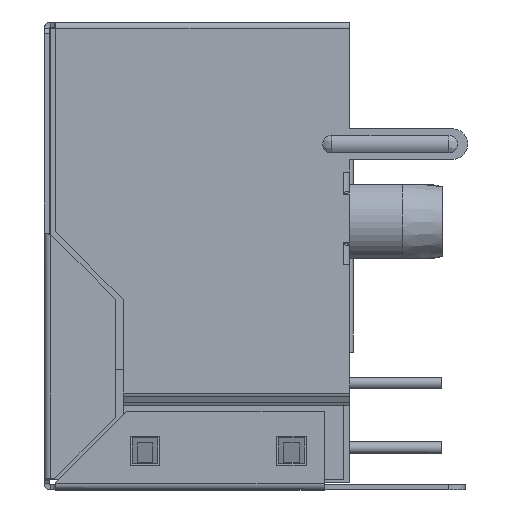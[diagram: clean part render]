
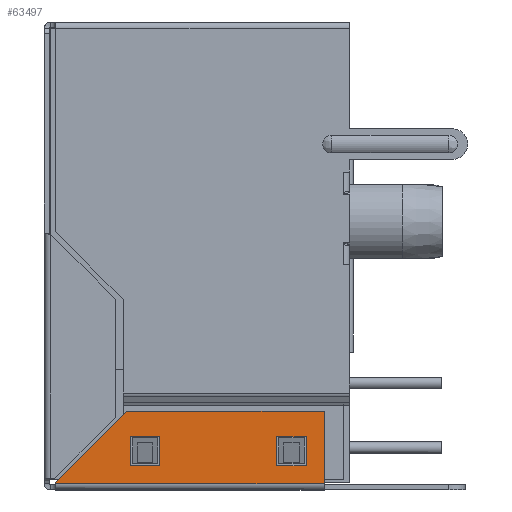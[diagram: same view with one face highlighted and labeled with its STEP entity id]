
A CAD part, left-side view. The second image highlights one B-rep face of the part: STEP entity #63497.
In plain terms, the highlighted planar face has unit normal (-1, 0, 0).
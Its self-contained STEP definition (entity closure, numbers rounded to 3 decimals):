
#437 = LINE ( 'NONE', #15104, #49154 ) ;
#512 = LINE ( 'NONE', #66749, #61142 ) ;
#621 = ORIENTED_EDGE ( 'NONE', *, *, #53207, .T. ) ;
#1085 = VECTOR ( 'NONE', #66073, 1000. ) ;
#2873 = DIRECTION ( 'NONE',  ( 0., 0.707, -0.707 ) ) ;
#2953 = DIRECTION ( 'NONE',  ( -1., 0., 0. ) ) ;
#3156 = CARTESIAN_POINT ( 'NONE',  ( -29.5, -3.145, -8.251 ) ) ;
#3959 = FACE_BOUND ( 'NONE', #29592, .T. ) ;
#4478 = VERTEX_POINT ( 'NONE', #22803 ) ;
#4897 = CARTESIAN_POINT ( 'NONE',  ( -29.5, 5.543, -8.951 ) ) ;
#5461 = LINE ( 'NONE', #19885, #10014 ) ;
#6989 = CARTESIAN_POINT ( 'NONE',  ( -29.5, 2.605, -8.251 ) ) ;
#9413 = ORIENTED_EDGE ( 'NONE', *, *, #43607, .T. ) ;
#9445 = ORIENTED_EDGE ( 'NONE', *, *, #21681, .F. ) ;
#9524 = CARTESIAN_POINT ( 'NONE',  ( -29.5, -5.211, -8.251 ) ) ;
#9581 = DIRECTION ( 'NONE',  ( 0., 0., -1. ) ) ;
#9731 = FACE_BOUND ( 'NONE', #72329, .T. ) ;
#10014 = VECTOR ( 'NONE', #50106, 1000. ) ;
#10704 = EDGE_CURVE ( 'NONE', #52799, #46683, #71140, .T. ) ;
#11021 = DIRECTION ( 'NONE',  ( 0., -1., 0. ) ) ;
#12224 = DIRECTION ( 'NONE',  ( 0., 1., 0. ) ) ;
#12351 = EDGE_CURVE ( 'NONE', #4478, #56018, #74597, .T. ) ;
#13058 = CARTESIAN_POINT ( 'NONE',  ( -29.5, -5., -8.951 ) ) ;
#15104 = CARTESIAN_POINT ( 'NONE',  ( -29.5, 2.605, -6.024 ) ) ;
#17156 = CARTESIAN_POINT ( 'NONE',  ( -29.5, -5., -6.024 ) ) ;
#17629 = CARTESIAN_POINT ( 'NONE',  ( -29.5, -5.211, -6.101 ) ) ;
#18092 = DIRECTION ( 'NONE',  ( 0., 0., -1. ) ) ;
#19599 = EDGE_LOOP ( 'NONE', ( #9445, #67479, #56314, #35001, #74691 ) ) ;
#19744 = ORIENTED_EDGE ( 'NONE', *, *, #12351, .T. ) ;
#19751 = VECTOR ( 'NONE', #55737, 1000. ) ;
#19885 = CARTESIAN_POINT ( 'NONE',  ( -29.5, -3.145, -6.024 ) ) ;
#20434 = PLANE ( 'NONE',  #64600 ) ;
#21681 = EDGE_CURVE ( 'NONE', #40056, #27289, #58455, .T. ) ;
#22007 = VERTEX_POINT ( 'NONE', #38034 ) ;
#22803 = CARTESIAN_POINT ( 'NONE',  ( -29.5, 1.455, -8.251 ) ) ;
#23699 = CARTESIAN_POINT ( 'NONE',  ( -29.5, -4.295, -6.024 ) ) ;
#25584 = EDGE_CURVE ( 'NONE', #36124, #22007, #41264, .T. ) ;
#25692 = VECTOR ( 'NONE', #2873, 1000. ) ;
#25715 = CARTESIAN_POINT ( 'NONE',  ( -29.5, 2.605, -7.101 ) ) ;
#27156 = ORIENTED_EDGE ( 'NONE', *, *, #10704, .T. ) ;
#27157 = CARTESIAN_POINT ( 'NONE',  ( -29.5, 2.75, -6.101 ) ) ;
#27182 = VECTOR ( 'NONE', #58178, 1000. ) ;
#27289 = VERTEX_POINT ( 'NONE', #4897 ) ;
#27569 = CARTESIAN_POINT ( 'NONE',  ( -29.5, -4.295, -8.251 ) ) ;
#28182 = LINE ( 'NONE', #17629, #66720 ) ;
#28316 = EDGE_CURVE ( 'NONE', #41098, #52799, #75872, .T. ) ;
#28424 = CARTESIAN_POINT ( 'NONE',  ( -29.5, -5.211, -7.101 ) ) ;
#28469 = CARTESIAN_POINT ( 'NONE',  ( -29.5, -4.295, -7.101 ) ) ;
#28540 = EDGE_CURVE ( 'NONE', #58259, #4478, #512, .T. ) ;
#28708 = VECTOR ( 'NONE', #67755, 1000. ) ;
#28829 = VECTOR ( 'NONE', #65834, 1000. ) ;
#29212 = EDGE_CURVE ( 'NONE', #56018, #69619, #437, .T. ) ;
#29592 = EDGE_LOOP ( 'NONE', ( #42643, #19744, #33779, #51431 ) ) ;
#30916 = EDGE_CURVE ( 'NONE', #22007, #27289, #72004, .T. ) ;
#32387 = VECTOR ( 'NONE', #11021, 1000. ) ;
#33779 = ORIENTED_EDGE ( 'NONE', *, *, #29212, .T. ) ;
#35001 = ORIENTED_EDGE ( 'NONE', *, *, #25584, .T. ) ;
#35769 = CARTESIAN_POINT ( 'NONE',  ( -29.5, -5., -6.101 ) ) ;
#36124 = VERTEX_POINT ( 'NONE', #27157 ) ;
#37723 = DIRECTION ( 'NONE',  ( 0., 0., -1. ) ) ;
#38034 = CARTESIAN_POINT ( 'NONE',  ( -29.5, 5.543, -8.894 ) ) ;
#38332 = CARTESIAN_POINT ( 'NONE',  ( -29.5, 1.455, -7.101 ) ) ;
#38780 = LINE ( 'NONE', #28424, #32387 ) ;
#40056 = VERTEX_POINT ( 'NONE', #13058 ) ;
#40466 = VERTEX_POINT ( 'NONE', #35769 ) ;
#40696 = VECTOR ( 'NONE', #9581, 1000. ) ;
#41098 = VERTEX_POINT ( 'NONE', #28469 ) ;
#41264 = LINE ( 'NONE', #60908, #25692 ) ;
#42643 = ORIENTED_EDGE ( 'NONE', *, *, #28540, .T. ) ;
#43607 = EDGE_CURVE ( 'NONE', #67095, #41098, #38780, .T. ) ;
#44680 = CARTESIAN_POINT ( 'NONE',  ( -29.5, 5.543, -6.024 ) ) ;
#46683 = VERTEX_POINT ( 'NONE', #3156 ) ;
#49154 = VECTOR ( 'NONE', #73624, 1000. ) ;
#50074 = CARTESIAN_POINT ( 'NONE',  ( -29.5, -5.211, -7.101 ) ) ;
#50106 = DIRECTION ( 'NONE',  ( 0., 0., 1. ) ) ;
#51431 = ORIENTED_EDGE ( 'NONE', *, *, #68142, .T. ) ;
#52799 = VERTEX_POINT ( 'NONE', #27569 ) ;
#53207 = EDGE_CURVE ( 'NONE', #46683, #67095, #5461, .T. ) ;
#55737 = DIRECTION ( 'NONE',  ( 0., 1., 0. ) ) ;
#56018 = VERTEX_POINT ( 'NONE', #6989 ) ;
#56314 = ORIENTED_EDGE ( 'NONE', *, *, #66004, .T. ) ;
#56558 = DIRECTION ( 'NONE',  ( 0., 0., 1. ) ) ;
#57935 = CARTESIAN_POINT ( 'NONE',  ( -29.5, -5., -8.951 ) ) ;
#58178 = DIRECTION ( 'NONE',  ( 0., 1., 0. ) ) ;
#58259 = VERTEX_POINT ( 'NONE', #38332 ) ;
#58455 = LINE ( 'NONE', #57935, #27182 ) ;
#58466 = ORIENTED_EDGE ( 'NONE', *, *, #28316, .T. ) ;
#60884 = LINE ( 'NONE', #50074, #28708 ) ;
#60908 = CARTESIAN_POINT ( 'NONE',  ( -29.5, 2.75, -6.101 ) ) ;
#60961 = CARTESIAN_POINT ( 'NONE',  ( -29.5, -5.211, -8.251 ) ) ;
#61114 = EDGE_CURVE ( 'NONE', #40056, #40466, #75729, .T. ) ;
#61142 = VECTOR ( 'NONE', #37723, 1000. ) ;
#61959 = CARTESIAN_POINT ( 'NONE',  ( -29.5, -5.211, -6.024 ) ) ;
#63497 = ADVANCED_FACE ( 'NONE', ( #3959, #9731, #69127 ), #20434, .T. ) ;
#64600 = AXIS2_PLACEMENT_3D ( 'NONE', #61959, #2953, #56558 ) ;
#65834 = DIRECTION ( 'NONE',  ( 0., 0., 1. ) ) ;
#66004 = EDGE_CURVE ( 'NONE', #40466, #36124, #28182, .T. ) ;
#66073 = DIRECTION ( 'NONE',  ( 0., 1., 0. ) ) ;
#66631 = VECTOR ( 'NONE', #18092, 1000. ) ;
#66720 = VECTOR ( 'NONE', #12224, 1000. ) ;
#66749 = CARTESIAN_POINT ( 'NONE',  ( -29.5, 1.455, -6.024 ) ) ;
#67095 = VERTEX_POINT ( 'NONE', #68233 ) ;
#67479 = ORIENTED_EDGE ( 'NONE', *, *, #61114, .T. ) ;
#67755 = DIRECTION ( 'NONE',  ( 0., -1., 0. ) ) ;
#68142 = EDGE_CURVE ( 'NONE', #69619, #58259, #60884, .T. ) ;
#68233 = CARTESIAN_POINT ( 'NONE',  ( -29.5, -3.145, -7.101 ) ) ;
#69127 = FACE_OUTER_BOUND ( 'NONE', #19599, .T. ) ;
#69619 = VERTEX_POINT ( 'NONE', #25715 ) ;
#71140 = LINE ( 'NONE', #9524, #19751 ) ;
#72004 = LINE ( 'NONE', #44680, #40696 ) ;
#72329 = EDGE_LOOP ( 'NONE', ( #58466, #27156, #621, #9413 ) ) ;
#73624 = DIRECTION ( 'NONE',  ( 0., 0., 1. ) ) ;
#74597 = LINE ( 'NONE', #60961, #1085 ) ;
#74691 = ORIENTED_EDGE ( 'NONE', *, *, #30916, .T. ) ;
#75729 = LINE ( 'NONE', #17156, #28829 ) ;
#75872 = LINE ( 'NONE', #23699, #66631 ) ;
